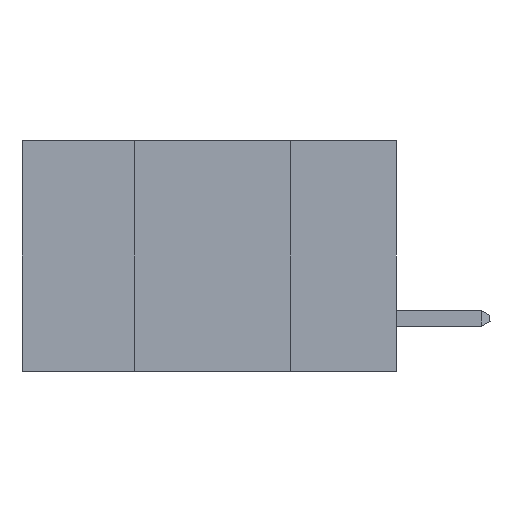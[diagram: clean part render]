
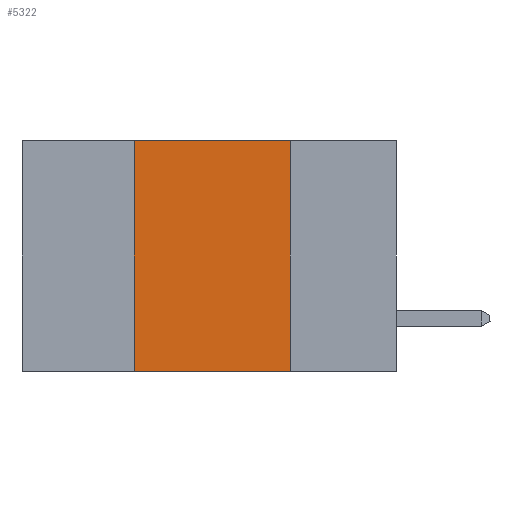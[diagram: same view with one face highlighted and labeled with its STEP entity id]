
A CAD part, left-side view. The second image highlights one B-rep face of the part: STEP entity #5322.
In plain terms, the highlighted planar face has unit normal (-1, 0, 0).
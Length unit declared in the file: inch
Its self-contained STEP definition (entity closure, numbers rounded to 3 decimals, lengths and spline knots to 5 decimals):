
#69 = EDGE_CURVE ( 'NONE', #20665, #14778, #7606, .T. ) ;
#949 = DIRECTION ( 'NONE',  ( 0., 0., 1. ) ) ;
#2110 = CARTESIAN_POINT ( 'NONE',  ( 0., 0.6, 0. ) ) ;
#2911 = CARTESIAN_POINT ( 'NONE',  ( 0., 0.6, 0. ) ) ;
#3125 = VECTOR ( 'NONE', #16263, 39.37008 ) ;
#3278 = VECTOR ( 'NONE', #949, 39.37008 ) ;
#3818 = ORIENTED_EDGE ( 'NONE', *, *, #17838, .F. ) ;
#3858 = VECTOR ( 'NONE', #13365, 39.37008 ) ;
#3903 = PLANE ( 'NONE',  #5179 ) ;
#4613 = CARTESIAN_POINT ( 'NONE',  ( 0., 0.42, -0.37 ) ) ;
#4974 = VERTEX_POINT ( 'NONE', #19710 ) ;
#5179 = AXIS2_PLACEMENT_3D ( 'NONE', #2911, #10728, #10630 ) ;
#5322 = ADVANCED_FACE ( 'NONE', ( #13164 ), #3903, .F. ) ;
#6584 = ORIENTED_EDGE ( 'NONE', *, *, #7938, .T. ) ;
#7019 = LINE ( 'NONE', #14126, #19619 ) ;
#7111 = CARTESIAN_POINT ( 'NONE',  ( 0., 0.42, 0. ) ) ;
#7153 = VERTEX_POINT ( 'NONE', #4613 ) ;
#7606 = LINE ( 'NONE', #2110, #3125 ) ;
#7938 = EDGE_CURVE ( 'NONE', #7153, #4974, #7019, .T. ) ;
#9148 = EDGE_LOOP ( 'NONE', ( #10933, #19856, #3818, #6584 ) ) ;
#10036 = CARTESIAN_POINT ( 'NONE',  ( 0., 0.17, 0. ) ) ;
#10630 = DIRECTION ( 'NONE',  ( 0., 0., -1. ) ) ;
#10728 = DIRECTION ( 'NONE',  ( 1., 0., 0. ) ) ;
#10933 = ORIENTED_EDGE ( 'NONE', *, *, #12403, .F. ) ;
#12403 = EDGE_CURVE ( 'NONE', #14778, #4974, #21398, .T. ) ;
#12741 = LINE ( 'NONE', #20860, #3278 ) ;
#13164 = FACE_OUTER_BOUND ( 'NONE', #9148, .T. ) ;
#13365 = DIRECTION ( 'NONE',  ( 0., 0., -1. ) ) ;
#13479 = CARTESIAN_POINT ( 'NONE',  ( 0., 0.17, 0. ) ) ;
#13872 = DIRECTION ( 'NONE',  ( 0., -1., 0. ) ) ;
#14126 = CARTESIAN_POINT ( 'NONE',  ( 0., 0.6, -0.37 ) ) ;
#14778 = VERTEX_POINT ( 'NONE', #13479 ) ;
#16263 = DIRECTION ( 'NONE',  ( 0., -1., 0. ) ) ;
#17838 = EDGE_CURVE ( 'NONE', #7153, #20665, #12741, .T. ) ;
#19619 = VECTOR ( 'NONE', #13872, 39.37008 ) ;
#19710 = CARTESIAN_POINT ( 'NONE',  ( 0., 0.17, -0.37 ) ) ;
#19856 = ORIENTED_EDGE ( 'NONE', *, *, #69, .F. ) ;
#20665 = VERTEX_POINT ( 'NONE', #7111 ) ;
#20860 = CARTESIAN_POINT ( 'NONE',  ( 0., 0.42, 0. ) ) ;
#21398 = LINE ( 'NONE', #10036, #3858 ) ;
